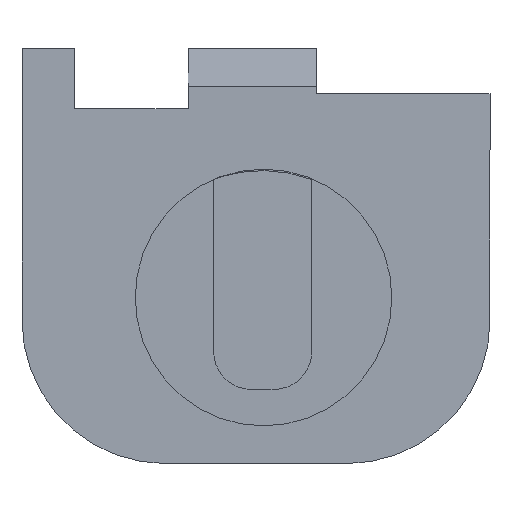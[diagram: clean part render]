
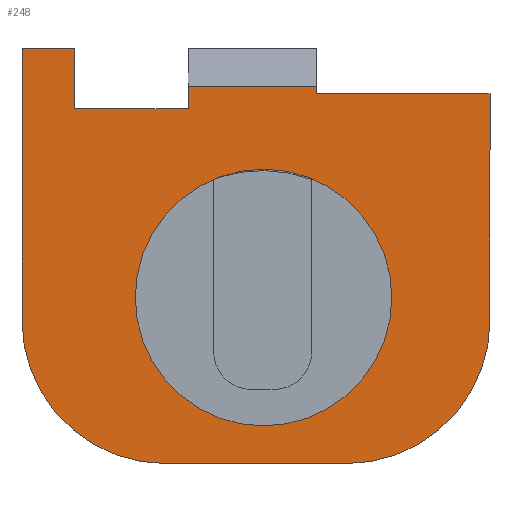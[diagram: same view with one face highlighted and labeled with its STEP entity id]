
A CAD part, front view. The second image highlights one B-rep face of the part: STEP entity #248.
In plain terms, the highlighted planar face has unit normal (0, -1, 0).
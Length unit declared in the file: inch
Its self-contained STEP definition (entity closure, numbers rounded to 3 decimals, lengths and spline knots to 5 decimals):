
#1 = AXIS2_PLACEMENT_3D ( 'NONE', #546, #143, #952 ) ;
#21 = CARTESIAN_POINT ( 'NONE',  ( -0.11302, 0., -0.33569 ) ) ;
#26 = VECTOR ( 'NONE', #960, 39.37008 ) ;
#36 = VERTEX_POINT ( 'NONE', #1011 ) ;
#46 = VECTOR ( 'NONE', #1041, 39.37008 ) ;
#49 = LINE ( 'NONE', #223, #964 ) ;
#52 = VERTEX_POINT ( 'NONE', #715 ) ;
#55 = CARTESIAN_POINT ( 'NONE',  ( 0., 0., 0.15431 ) ) ;
#57 = EDGE_CURVE ( 'NONE', #470, #52, #474, .T. ) ;
#62 = VECTOR ( 'NONE', #1039, 39.37008 ) ;
#64 = DIRECTION ( 'NONE',  ( 0., 0., 1. ) ) ;
#68 = EDGE_CURVE ( 'NONE', #108, #299, #475, .T. ) ;
#72 = LINE ( 'NONE', #974, #142 ) ;
#77 = FACE_OUTER_BOUND ( 'NONE', #520, .T. ) ;
#80 = CARTESIAN_POINT ( 'NONE',  ( 0.12698, 0., -0.14569 ) ) ;
#88 = CARTESIAN_POINT ( 'NONE',  ( -0.08302, 0., 0.16414 ) ) ;
#95 = EDGE_CURVE ( 'NONE', #299, #108, #664, .T. ) ;
#108 = VERTEX_POINT ( 'NONE', #484 ) ;
#138 = CARTESIAN_POINT ( 'NONE',  ( 0.01698, 0., -0.11569 ) ) ;
#140 = LINE ( 'NONE', #55, #662 ) ;
#142 = VECTOR ( 'NONE', #249, 39.37008 ) ;
#143 = DIRECTION ( 'NONE',  ( 0., 1., 0. ) ) ;
#148 = CARTESIAN_POINT ( 'NONE',  ( 0.31698, 0., 0.15431 ) ) ;
#152 = EDGE_CURVE ( 'NONE', #485, #52, #140, .T. ) ;
#154 = LINE ( 'NONE', #730, #46 ) ;
#159 = EDGE_CURVE ( 'NONE', #625, #36, #353, .T. ) ;
#168 = ORIENTED_EDGE ( 'NONE', *, *, #341, .F. ) ;
#171 = VECTOR ( 'NONE', #782, 39.37008 ) ;
#195 = CARTESIAN_POINT ( 'NONE',  ( -0.23302, 0., 0.21431 ) ) ;
#208 = CARTESIAN_POINT ( 'NONE',  ( -0.30302, 0., 0. ) ) ;
#223 = CARTESIAN_POINT ( 'NONE',  ( -0.09, 0., 0.16414 ) ) ;
#233 = VERTEX_POINT ( 'NONE', #566 ) ;
#237 = CARTESIAN_POINT ( 'NONE',  ( 0.31698, 0., 0. ) ) ;
#238 = CARTESIAN_POINT ( 'NONE',  ( 0.08698, 0., 0.16414 ) ) ;
#248 = ADVANCED_FACE ( 'NONE', ( #489, #77 ), #441, .F. ) ;
#249 = DIRECTION ( 'NONE',  ( -1., 0., 0. ) ) ;
#266 = EDGE_CURVE ( 'NONE', #508, #575, #72, .T. ) ;
#273 = DIRECTION ( 'NONE',  ( 0., 1., 0. ) ) ;
#284 = AXIS2_PLACEMENT_3D ( 'NONE', #749, #273, #671 ) ;
#299 = VERTEX_POINT ( 'NONE', #366 ) ;
#300 = EDGE_CURVE ( 'NONE', #508, #579, #732, .T. ) ;
#341 = EDGE_CURVE ( 'NONE', #390, #470, #49, .T. ) ;
#342 = DIRECTION ( 'NONE',  ( 0., 0., 1. ) ) ;
#346 = EDGE_CURVE ( 'NONE', #390, #1003, #629, .T. ) ;
#353 = CIRCLE ( 'NONE', #944, 0.19 ) ;
#366 = CARTESIAN_POINT ( 'NONE',  ( 0.01698, 0., 0.05431 ) ) ;
#372 = ORIENTED_EDGE ( 'NONE', *, *, #300, .F. ) ;
#378 = CIRCLE ( 'NONE', #427, 0.19 ) ;
#385 = ORIENTED_EDGE ( 'NONE', *, *, #159, .F. ) ;
#390 = VERTEX_POINT ( 'NONE', #88 ) ;
#427 = AXIS2_PLACEMENT_3D ( 'NONE', #80, #584, #342 ) ;
#429 = ORIENTED_EDGE ( 'NONE', *, *, #856, .T. ) ;
#441 = PLANE ( 'NONE',  #284 ) ;
#447 = ORIENTED_EDGE ( 'NONE', *, *, #894, .F. ) ;
#468 = DIRECTION ( 'NONE',  ( 1., 0., 0. ) ) ;
#470 = VERTEX_POINT ( 'NONE', #238 ) ;
#474 = LINE ( 'NONE', #634, #26 ) ;
#475 = CIRCLE ( 'NONE', #904, 0.17 ) ;
#480 = DIRECTION ( 'NONE',  ( -1., 0., 0. ) ) ;
#484 = CARTESIAN_POINT ( 'NONE',  ( 0.01698, 0., -0.28569 ) ) ;
#485 = VERTEX_POINT ( 'NONE', #148 ) ;
#488 = EDGE_CURVE ( 'NONE', #625, #233, #154, .T. ) ;
#489 = FACE_BOUND ( 'NONE', #681, .T. ) ;
#501 = EDGE_CURVE ( 'NONE', #564, #233, #378, .T. ) ;
#508 = VERTEX_POINT ( 'NONE', #195 ) ;
#516 = ORIENTED_EDGE ( 'NONE', *, *, #68, .T. ) ;
#520 = EDGE_LOOP ( 'NONE', ( #755, #168, #885, #539, #372, #648, #447, #385, #852, #845, #429, #981 ) ) ;
#522 = VECTOR ( 'NONE', #1032, 39.37008 ) ;
#523 = DIRECTION ( 'NONE',  ( 0., 0., 1. ) ) ;
#535 = CARTESIAN_POINT ( 'NONE',  ( -0.30302, 0., 0.21431 ) ) ;
#539 = ORIENTED_EDGE ( 'NONE', *, *, #565, .F. ) ;
#540 = LINE ( 'NONE', #581, #522 ) ;
#546 = CARTESIAN_POINT ( 'NONE',  ( 0.01698, 0., -0.11569 ) ) ;
#564 = VERTEX_POINT ( 'NONE', #880 ) ;
#565 = EDGE_CURVE ( 'NONE', #579, #1003, #540, .T. ) ;
#566 = CARTESIAN_POINT ( 'NONE',  ( 0.12698, 0., -0.33569 ) ) ;
#575 = VERTEX_POINT ( 'NONE', #535 ) ;
#579 = VERTEX_POINT ( 'NONE', #911 ) ;
#581 = CARTESIAN_POINT ( 'NONE',  ( 0., 0., 0.13431 ) ) ;
#584 = DIRECTION ( 'NONE',  ( 0., 1., 0. ) ) ;
#586 = VECTOR ( 'NONE', #523, 39.37008 ) ;
#587 = ORIENTED_EDGE ( 'NONE', *, *, #95, .T. ) ;
#611 = LINE ( 'NONE', #208, #586 ) ;
#625 = VERTEX_POINT ( 'NONE', #21 ) ;
#629 = LINE ( 'NONE', #770, #171 ) ;
#634 = CARTESIAN_POINT ( 'NONE',  ( 0.08698, 0., 0. ) ) ;
#648 = ORIENTED_EDGE ( 'NONE', *, *, #266, .T. ) ;
#650 = VECTOR ( 'NONE', #677, 39.37008 ) ;
#662 = VECTOR ( 'NONE', #480, 39.37008 ) ;
#664 = CIRCLE ( 'NONE', #1, 0.17 ) ;
#671 = DIRECTION ( 'NONE',  ( 0., 0., 1. ) ) ;
#677 = DIRECTION ( 'NONE',  ( 0., 0., -1. ) ) ;
#679 = CARTESIAN_POINT ( 'NONE',  ( -0.08302, 0., 0.13431 ) ) ;
#681 = EDGE_LOOP ( 'NONE', ( #516, #587 ) ) ;
#715 = CARTESIAN_POINT ( 'NONE',  ( 0.08698, 0., 0.15431 ) ) ;
#730 = CARTESIAN_POINT ( 'NONE',  ( 0., 0., -0.33569 ) ) ;
#732 = LINE ( 'NONE', #1000, #650 ) ;
#749 = CARTESIAN_POINT ( 'NONE',  ( 0., 0., 0. ) ) ;
#755 = ORIENTED_EDGE ( 'NONE', *, *, #57, .F. ) ;
#770 = CARTESIAN_POINT ( 'NONE',  ( -0.08302, 0., 0. ) ) ;
#782 = DIRECTION ( 'NONE',  ( 0., 0., -1. ) ) ;
#789 = DIRECTION ( 'NONE',  ( 0., 1., 0. ) ) ;
#794 = DIRECTION ( 'NONE',  ( 0., 1., 0. ) ) ;
#801 = CARTESIAN_POINT ( 'NONE',  ( -0.11302, 0., -0.14569 ) ) ;
#845 = ORIENTED_EDGE ( 'NONE', *, *, #501, .F. ) ;
#852 = ORIENTED_EDGE ( 'NONE', *, *, #488, .T. ) ;
#856 = EDGE_CURVE ( 'NONE', #564, #485, #866, .T. ) ;
#866 = LINE ( 'NONE', #237, #62 ) ;
#880 = CARTESIAN_POINT ( 'NONE',  ( 0.31698, 0., -0.14569 ) ) ;
#885 = ORIENTED_EDGE ( 'NONE', *, *, #346, .T. ) ;
#894 = EDGE_CURVE ( 'NONE', #36, #575, #611, .T. ) ;
#904 = AXIS2_PLACEMENT_3D ( 'NONE', #138, #794, #64 ) ;
#911 = CARTESIAN_POINT ( 'NONE',  ( -0.23302, 0., 0.13431 ) ) ;
#944 = AXIS2_PLACEMENT_3D ( 'NONE', #801, #789, #962 ) ;
#952 = DIRECTION ( 'NONE',  ( 0., 0., 1. ) ) ;
#960 = DIRECTION ( 'NONE',  ( 0., 0., -1. ) ) ;
#962 = DIRECTION ( 'NONE',  ( 0., 0., 1. ) ) ;
#964 = VECTOR ( 'NONE', #468, 39.37008 ) ;
#974 = CARTESIAN_POINT ( 'NONE',  ( 0., 0., 0.21431 ) ) ;
#981 = ORIENTED_EDGE ( 'NONE', *, *, #152, .T. ) ;
#1000 = CARTESIAN_POINT ( 'NONE',  ( -0.23302, 0., 0. ) ) ;
#1003 = VERTEX_POINT ( 'NONE', #679 ) ;
#1011 = CARTESIAN_POINT ( 'NONE',  ( -0.30302, 0., -0.14569 ) ) ;
#1032 = DIRECTION ( 'NONE',  ( 1., 0., 0. ) ) ;
#1039 = DIRECTION ( 'NONE',  ( 0., 0., 1. ) ) ;
#1041 = DIRECTION ( 'NONE',  ( 1., 0., 0. ) ) ;
